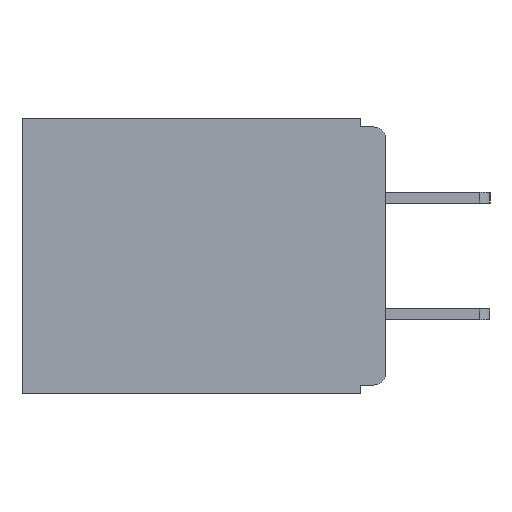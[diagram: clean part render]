
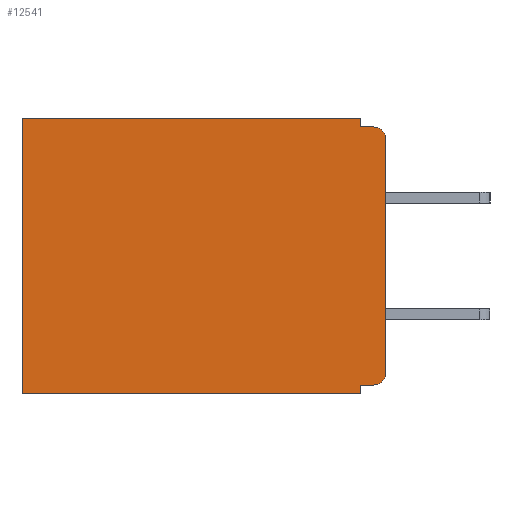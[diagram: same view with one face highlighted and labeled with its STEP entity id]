
A CAD part, left-side view. The second image highlights one B-rep face of the part: STEP entity #12541.
In plain terms, the highlighted planar face has unit normal (-1, 0, 0).
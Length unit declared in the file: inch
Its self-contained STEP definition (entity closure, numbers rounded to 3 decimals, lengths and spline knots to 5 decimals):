
#393 = AXIS2_PLACEMENT_3D ( 'NONE', #17593, #17683, #3143 ) ;
#1630 = VECTOR ( 'NONE', #20147, 39.37008 ) ;
#2102 = VERTEX_POINT ( 'NONE', #3268 ) ;
#2554 = LINE ( 'NONE', #17628, #8236 ) ;
#2622 = LINE ( 'NONE', #27053, #14805 ) ;
#2647 = VERTEX_POINT ( 'NONE', #24376 ) ;
#2909 = CARTESIAN_POINT ( 'NONE',  ( 0.3, 0.015, -0.025 ) ) ;
#2979 = AXIS2_PLACEMENT_3D ( 'NONE', #23606, #9194, #26023 ) ;
#3143 = DIRECTION ( 'NONE',  ( 0., 0., -1. ) ) ;
#3268 = CARTESIAN_POINT ( 'NONE',  ( 0.3, 0.437, -0.33 ) ) ;
#3697 = ORIENTED_EDGE ( 'NONE', *, *, #22491, .T. ) ;
#4216 = VECTOR ( 'NONE', #15475, 39.37008 ) ;
#5056 = AXIS2_PLACEMENT_3D ( 'NONE', #2909, #5507, #5442 ) ;
#5311 = VECTOR ( 'NONE', #13676, 39.37008 ) ;
#5442 = DIRECTION ( 'NONE',  ( 0., 0., -1. ) ) ;
#5507 = DIRECTION ( 'NONE',  ( -1., 0., 0. ) ) ;
#5521 = DIRECTION ( 'NONE',  ( 0., -1., 0. ) ) ;
#5661 = EDGE_CURVE ( 'NONE', #24373, #28626, #14644, .T. ) ;
#6066 = EDGE_CURVE ( 'NONE', #24373, #9328, #9648, .T. ) ;
#7052 = EDGE_CURVE ( 'NONE', #12356, #2647, #13764, .T. ) ;
#7787 = DIRECTION ( 'NONE',  ( 0., 1., 0. ) ) ;
#8177 = ORIENTED_EDGE ( 'NONE', *, *, #30023, .F. ) ;
#8195 = DIRECTION ( 'NONE',  ( 0., 0., -1. ) ) ;
#8236 = VECTOR ( 'NONE', #5521, 39.37008 ) ;
#8543 = CARTESIAN_POINT ( 'NONE',  ( 0.3, 0.031, -0.33 ) ) ;
#8631 = ORIENTED_EDGE ( 'NONE', *, *, #23249, .F. ) ;
#8731 = DIRECTION ( 'NONE',  ( 0., 0., -1. ) ) ;
#8748 = VERTEX_POINT ( 'NONE', #10695 ) ;
#8790 = CARTESIAN_POINT ( 'NONE',  ( 0.3, 0., -0.33 ) ) ;
#8827 = VECTOR ( 'NONE', #8731, 39.37008 ) ;
#8879 = EDGE_CURVE ( 'NONE', #22602, #2102, #18223, .T. ) ;
#9194 = DIRECTION ( 'NONE',  ( -1., 0., 0. ) ) ;
#9328 = VERTEX_POINT ( 'NONE', #29677 ) ;
#9648 = CIRCLE ( 'NONE', #5056, 0.015 ) ;
#9847 = CARTESIAN_POINT ( 'NONE',  ( 0.3, 0.031, -0.01 ) ) ;
#10695 = CARTESIAN_POINT ( 'NONE',  ( 0.3, 0.437, 0. ) ) ;
#12128 = CARTESIAN_POINT ( 'NONE',  ( 0.3, 0., -0.305 ) ) ;
#12356 = VERTEX_POINT ( 'NONE', #28884 ) ;
#12541 = ADVANCED_FACE ( 'NONE', ( #30122 ), #15182, .F. ) ;
#12772 = ORIENTED_EDGE ( 'NONE', *, *, #6066, .T. ) ;
#12846 = EDGE_CURVE ( 'NONE', #12356, #28626, #29417, .T. ) ;
#13134 = EDGE_CURVE ( 'NONE', #20123, #8748, #2622, .T. ) ;
#13676 = DIRECTION ( 'NONE',  ( 0., 1., 0. ) ) ;
#13764 = LINE ( 'NONE', #17668, #1630 ) ;
#14557 = LINE ( 'NONE', #30387, #8827 ) ;
#14644 = LINE ( 'NONE', #20370, #27343 ) ;
#14805 = VECTOR ( 'NONE', #7787, 39.37008 ) ;
#15182 = PLANE ( 'NONE',  #393 ) ;
#15475 = DIRECTION ( 'NONE',  ( 0., 0., -1. ) ) ;
#15828 = ORIENTED_EDGE ( 'NONE', *, *, #13134, .T. ) ;
#17593 = CARTESIAN_POINT ( 'NONE',  ( 0.3, 0., -0.33 ) ) ;
#17628 = CARTESIAN_POINT ( 'NONE',  ( 0.3, 0., -0.01 ) ) ;
#17668 = CARTESIAN_POINT ( 'NONE',  ( 0.3, 0., -0.32 ) ) ;
#17683 = DIRECTION ( 'NONE',  ( 1., 0., 0. ) ) ;
#17783 = CARTESIAN_POINT ( 'NONE',  ( 0.3, 0., -0.025 ) ) ;
#18026 = ORIENTED_EDGE ( 'NONE', *, *, #5661, .F. ) ;
#18205 = EDGE_CURVE ( 'NONE', #29307, #9328, #2554, .T. ) ;
#18223 = LINE ( 'NONE', #8790, #5311 ) ;
#20123 = VERTEX_POINT ( 'NONE', #29208 ) ;
#20147 = DIRECTION ( 'NONE',  ( 0., 1., 0. ) ) ;
#20223 = ORIENTED_EDGE ( 'NONE', *, *, #18205, .F. ) ;
#20370 = CARTESIAN_POINT ( 'NONE',  ( 0.3, 0., -0.33 ) ) ;
#22491 = EDGE_CURVE ( 'NONE', #8748, #2102, #29840, .T. ) ;
#22602 = VERTEX_POINT ( 'NONE', #8543 ) ;
#23249 = EDGE_CURVE ( 'NONE', #2647, #22602, #14557, .T. ) ;
#23453 = LINE ( 'NONE', #27465, #29826 ) ;
#23606 = CARTESIAN_POINT ( 'NONE',  ( 0.3, 0.015, -0.305 ) ) ;
#23776 = ORIENTED_EDGE ( 'NONE', *, *, #7052, .F. ) ;
#24373 = VERTEX_POINT ( 'NONE', #17783 ) ;
#24376 = CARTESIAN_POINT ( 'NONE',  ( 0.3, 0.031, -0.32 ) ) ;
#25771 = ORIENTED_EDGE ( 'NONE', *, *, #12846, .T. ) ;
#25812 = ORIENTED_EDGE ( 'NONE', *, *, #8879, .F. ) ;
#26023 = DIRECTION ( 'NONE',  ( 0., 0., -1. ) ) ;
#27053 = CARTESIAN_POINT ( 'NONE',  ( 0.3, 0., 0. ) ) ;
#27343 = VECTOR ( 'NONE', #31152, 39.37008 ) ;
#27378 = CARTESIAN_POINT ( 'NONE',  ( 0.3, 0.437, -0.33 ) ) ;
#27465 = CARTESIAN_POINT ( 'NONE',  ( 0.3, 0.031, 0. ) ) ;
#28626 = VERTEX_POINT ( 'NONE', #12128 ) ;
#28884 = CARTESIAN_POINT ( 'NONE',  ( 0.3, 0.015, -0.32 ) ) ;
#29208 = CARTESIAN_POINT ( 'NONE',  ( 0.3, 0.031, 0. ) ) ;
#29307 = VERTEX_POINT ( 'NONE', #9847 ) ;
#29417 = CIRCLE ( 'NONE', #2979, 0.015 ) ;
#29677 = CARTESIAN_POINT ( 'NONE',  ( 0.3, 0.015, -0.01 ) ) ;
#29826 = VECTOR ( 'NONE', #8195, 39.37008 ) ;
#29840 = LINE ( 'NONE', #27378, #4216 ) ;
#29989 = EDGE_LOOP ( 'NONE', ( #18026, #12772, #20223, #8177, #15828, #3697, #25812, #8631, #23776, #25771 ) ) ;
#30023 = EDGE_CURVE ( 'NONE', #20123, #29307, #23453, .T. ) ;
#30122 = FACE_OUTER_BOUND ( 'NONE', #29989, .T. ) ;
#30387 = CARTESIAN_POINT ( 'NONE',  ( 0.3, 0.031, -0.33 ) ) ;
#31152 = DIRECTION ( 'NONE',  ( 0., 0., -1. ) ) ;
